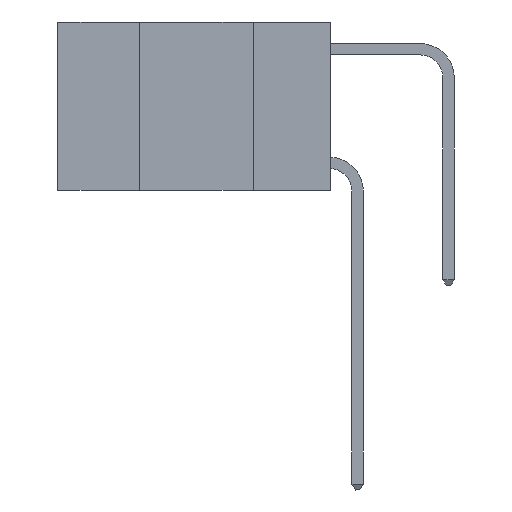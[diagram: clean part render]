
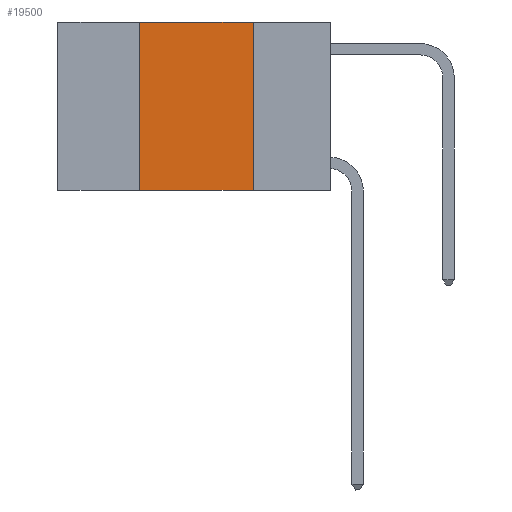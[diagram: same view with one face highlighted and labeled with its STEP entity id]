
A CAD part, left-side view. The second image highlights one B-rep face of the part: STEP entity #19500.
In plain terms, the highlighted planar face has unit normal (-1, 0, 0).
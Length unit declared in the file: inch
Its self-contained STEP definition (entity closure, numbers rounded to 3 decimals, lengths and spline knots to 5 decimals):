
#421 = FACE_OUTER_BOUND ( 'NONE', #29284, .T. ) ;
#1043 = CARTESIAN_POINT ( 'NONE',  ( 0., 0.42, 0. ) ) ;
#1346 = CARTESIAN_POINT ( 'NONE',  ( 0., 0.17, 0. ) ) ;
#1396 = LINE ( 'NONE', #5434, #2192 ) ;
#1851 = VECTOR ( 'NONE', #21576, 39.37008 ) ;
#2192 = VECTOR ( 'NONE', #7961, 39.37008 ) ;
#2571 = EDGE_CURVE ( 'NONE', #23733, #21735, #1396, .T. ) ;
#5098 = PLANE ( 'NONE',  #26821 ) ;
#5434 = CARTESIAN_POINT ( 'NONE',  ( 0., 0.6, -0.37 ) ) ;
#5597 = CARTESIAN_POINT ( 'NONE',  ( 0., 0.42, -0.37 ) ) ;
#6424 = CARTESIAN_POINT ( 'NONE',  ( 0., 0.6, 0. ) ) ;
#6681 = CARTESIAN_POINT ( 'NONE',  ( 0., 0.17, 0. ) ) ;
#7025 = VECTOR ( 'NONE', #8549, 39.37008 ) ;
#7123 = CARTESIAN_POINT ( 'NONE',  ( 0., 0.42, 0. ) ) ;
#7537 = CARTESIAN_POINT ( 'NONE',  ( 0., 0.17, -0.37 ) ) ;
#7629 = DIRECTION ( 'NONE',  ( 0., 0., -1. ) ) ;
#7961 = DIRECTION ( 'NONE',  ( 0., -1., 0. ) ) ;
#8549 = DIRECTION ( 'NONE',  ( 0., 0., 1. ) ) ;
#9207 = DIRECTION ( 'NONE',  ( 0., 0., -1. ) ) ;
#9403 = LINE ( 'NONE', #6681, #22072 ) ;
#10187 = ORIENTED_EDGE ( 'NONE', *, *, #21337, .F. ) ;
#15277 = LINE ( 'NONE', #6424, #1851 ) ;
#16755 = VERTEX_POINT ( 'NONE', #1346 ) ;
#19500 = ADVANCED_FACE ( 'NONE', ( #421 ), #5098, .F. ) ;
#21285 = ORIENTED_EDGE ( 'NONE', *, *, #31082, .F. ) ;
#21337 = EDGE_CURVE ( 'NONE', #23733, #29260, #27923, .T. ) ;
#21576 = DIRECTION ( 'NONE',  ( 0., -1., 0. ) ) ;
#21735 = VERTEX_POINT ( 'NONE', #7537 ) ;
#22067 = ORIENTED_EDGE ( 'NONE', *, *, #31735, .F. ) ;
#22072 = VECTOR ( 'NONE', #9207, 39.37008 ) ;
#22773 = DIRECTION ( 'NONE',  ( 1., 0., 0. ) ) ;
#23733 = VERTEX_POINT ( 'NONE', #5597 ) ;
#26821 = AXIS2_PLACEMENT_3D ( 'NONE', #30230, #22773, #7629 ) ;
#27923 = LINE ( 'NONE', #1043, #7025 ) ;
#29260 = VERTEX_POINT ( 'NONE', #7123 ) ;
#29284 = EDGE_LOOP ( 'NONE', ( #21285, #22067, #10187, #30321 ) ) ;
#30230 = CARTESIAN_POINT ( 'NONE',  ( 0., 0.6, 0. ) ) ;
#30321 = ORIENTED_EDGE ( 'NONE', *, *, #2571, .T. ) ;
#31082 = EDGE_CURVE ( 'NONE', #16755, #21735, #9403, .T. ) ;
#31735 = EDGE_CURVE ( 'NONE', #29260, #16755, #15277, .T. ) ;
